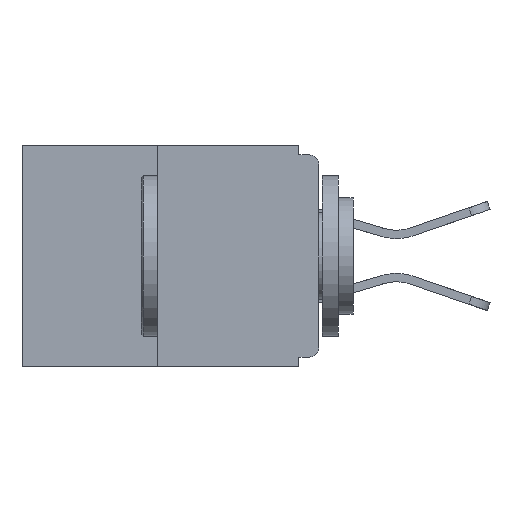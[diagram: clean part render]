
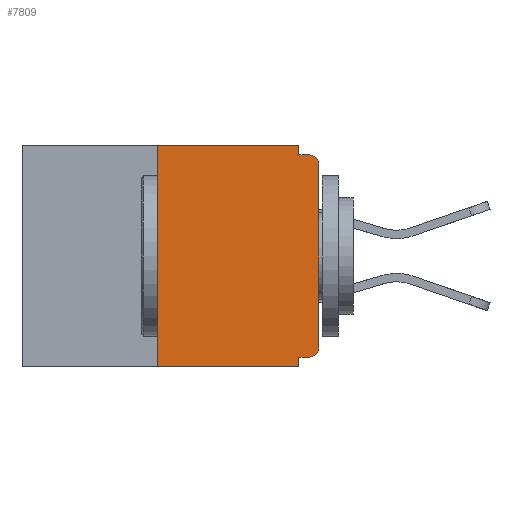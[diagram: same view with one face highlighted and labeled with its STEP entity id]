
A CAD part, left-side view. The second image highlights one B-rep face of the part: STEP entity #7809.
In plain terms, the highlighted planar face has unit normal (-1, 0, 0).
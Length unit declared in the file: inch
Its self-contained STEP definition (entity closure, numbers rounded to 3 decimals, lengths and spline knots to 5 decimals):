
#391 = DIRECTION ( 'NONE',  ( 0., -1., 0. ) ) ;
#411 = VECTOR ( 'NONE', #391, 39.37008 ) ;
#1763 = VERTEX_POINT ( 'NONE', #17021 ) ;
#2031 = CARTESIAN_POINT ( 'NONE',  ( 0., 0.015, -0.313 ) ) ;
#2103 = DIRECTION ( 'NONE',  ( 0., 0., 1. ) ) ;
#2507 = AXIS2_PLACEMENT_3D ( 'NONE', #2031, #16916, #10235 ) ;
#2935 = VERTEX_POINT ( 'NONE', #12909 ) ;
#2980 = CARTESIAN_POINT ( 'NONE',  ( 0., 0.031, -0.015 ) ) ;
#3116 = VECTOR ( 'NONE', #6594, 39.37008 ) ;
#3355 = EDGE_CURVE ( 'NONE', #2935, #6996, #9902, .T. ) ;
#3390 = VECTOR ( 'NONE', #12480, 39.37008 ) ;
#3739 = CARTESIAN_POINT ( 'NONE',  ( 0., 0.031, -0.343 ) ) ;
#3840 = CARTESIAN_POINT ( 'NONE',  ( 0., 0., 0. ) ) ;
#4443 = DIRECTION ( 'NONE',  ( 0., -1., 0. ) ) ;
#4661 = CARTESIAN_POINT ( 'NONE',  ( 0., 0.015, -0.03 ) ) ;
#4857 = AXIS2_PLACEMENT_3D ( 'NONE', #7709, #17078, #15802 ) ;
#4864 = CARTESIAN_POINT ( 'NONE',  ( 0., 0., -0.313 ) ) ;
#5045 = ORIENTED_EDGE ( 'NONE', *, *, #16976, .T. ) ;
#5208 = ORIENTED_EDGE ( 'NONE', *, *, #11124, .F. ) ;
#5465 = CARTESIAN_POINT ( 'NONE',  ( 0., 0.031, 0. ) ) ;
#5549 = VERTEX_POINT ( 'NONE', #4864 ) ;
#5625 = AXIS2_PLACEMENT_3D ( 'NONE', #4661, #9992, #8762 ) ;
#5684 = LINE ( 'NONE', #8951, #8833 ) ;
#5747 = CIRCLE ( 'NONE', #5625, 0.015 ) ;
#5835 = CARTESIAN_POINT ( 'NONE',  ( 0., 0.46, 0. ) ) ;
#5891 = CARTESIAN_POINT ( 'NONE',  ( 0., 0., -0.015 ) ) ;
#5989 = ORIENTED_EDGE ( 'NONE', *, *, #15294, .T. ) ;
#6482 = ORIENTED_EDGE ( 'NONE', *, *, #12952, .F. ) ;
#6594 = DIRECTION ( 'NONE',  ( 0., 0., -1. ) ) ;
#6836 = ORIENTED_EDGE ( 'NONE', *, *, #3355, .F. ) ;
#6996 = VERTEX_POINT ( 'NONE', #11893 ) ;
#7324 = VERTEX_POINT ( 'NONE', #11847 ) ;
#7512 = ORIENTED_EDGE ( 'NONE', *, *, #16741, .T. ) ;
#7709 = CARTESIAN_POINT ( 'NONE',  ( 0., 0.46, 0. ) ) ;
#7726 = VERTEX_POINT ( 'NONE', #14054 ) ;
#7809 = ADVANCED_FACE ( 'NONE', ( #8801 ), #14388, .F. ) ;
#8096 = VECTOR ( 'NONE', #4443, 39.37008 ) ;
#8340 = EDGE_CURVE ( 'NONE', #10479, #1763, #10663, .T. ) ;
#8451 = CARTESIAN_POINT ( 'NONE',  ( 0., 0.46, -0.343 ) ) ;
#8762 = DIRECTION ( 'NONE',  ( 0., 0., -1. ) ) ;
#8801 = FACE_OUTER_BOUND ( 'NONE', #10194, .T. ) ;
#8833 = VECTOR ( 'NONE', #12781, 39.37008 ) ;
#8951 = CARTESIAN_POINT ( 'NONE',  ( 0., 0., -0.328 ) ) ;
#9400 = ORIENTED_EDGE ( 'NONE', *, *, #8340, .F. ) ;
#9679 = CIRCLE ( 'NONE', #2507, 0.015 ) ;
#9817 = ORIENTED_EDGE ( 'NONE', *, *, #11422, .T. ) ;
#9902 = LINE ( 'NONE', #5835, #3390 ) ;
#9992 = DIRECTION ( 'NONE',  ( -1., 0., 0. ) ) ;
#10194 = EDGE_LOOP ( 'NONE', ( #6836, #5208, #7512, #9400, #12667, #5045, #9817, #5989, #6482, #14224 ) ) ;
#10235 = DIRECTION ( 'NONE',  ( 0., 0., -1. ) ) ;
#10479 = VERTEX_POINT ( 'NONE', #13318 ) ;
#10550 = VECTOR ( 'NONE', #13100, 39.37008 ) ;
#10663 = LINE ( 'NONE', #3739, #3116 ) ;
#10986 = VECTOR ( 'NONE', #2103, 39.37008 ) ;
#11124 = EDGE_CURVE ( 'NONE', #16109, #2935, #12472, .T. ) ;
#11422 = EDGE_CURVE ( 'NONE', #5549, #7726, #13708, .T. ) ;
#11847 = CARTESIAN_POINT ( 'NONE',  ( 0., 0.015, -0.328 ) ) ;
#11893 = CARTESIAN_POINT ( 'NONE',  ( 0., 0.031, 0. ) ) ;
#12183 = CARTESIAN_POINT ( 'NONE',  ( 0., 0.015, -0.015 ) ) ;
#12305 = LINE ( 'NONE', #5891, #8096 ) ;
#12472 = LINE ( 'NONE', #12854, #10986 ) ;
#12480 = DIRECTION ( 'NONE',  ( 0., -1., 0. ) ) ;
#12667 = ORIENTED_EDGE ( 'NONE', *, *, #16999, .F. ) ;
#12781 = DIRECTION ( 'NONE',  ( 0., 1., 0. ) ) ;
#12854 = CARTESIAN_POINT ( 'NONE',  ( 0., 0.25, 0. ) ) ;
#12909 = CARTESIAN_POINT ( 'NONE',  ( 0., 0.25, 0. ) ) ;
#12952 = EDGE_CURVE ( 'NONE', #13356, #13677, #12305, .T. ) ;
#13100 = DIRECTION ( 'NONE',  ( 0., 0., 1. ) ) ;
#13318 = CARTESIAN_POINT ( 'NONE',  ( 0., 0.031, -0.328 ) ) ;
#13356 = VERTEX_POINT ( 'NONE', #2980 ) ;
#13677 = VERTEX_POINT ( 'NONE', #12183 ) ;
#13708 = LINE ( 'NONE', #3840, #10550 ) ;
#14054 = CARTESIAN_POINT ( 'NONE',  ( 0., 0., -0.03 ) ) ;
#14224 = ORIENTED_EDGE ( 'NONE', *, *, #15774, .F. ) ;
#14388 = PLANE ( 'NONE',  #4857 ) ;
#14742 = LINE ( 'NONE', #5465, #15593 ) ;
#14847 = DIRECTION ( 'NONE',  ( 0., 0., -1. ) ) ;
#15294 = EDGE_CURVE ( 'NONE', #7726, #13677, #5747, .T. ) ;
#15593 = VECTOR ( 'NONE', #14847, 39.37008 ) ;
#15774 = EDGE_CURVE ( 'NONE', #6996, #13356, #14742, .T. ) ;
#15802 = DIRECTION ( 'NONE',  ( 0., 0., -1. ) ) ;
#16060 = CARTESIAN_POINT ( 'NONE',  ( 0., 0.25, -0.343 ) ) ;
#16109 = VERTEX_POINT ( 'NONE', #16060 ) ;
#16741 = EDGE_CURVE ( 'NONE', #16109, #1763, #16811, .T. ) ;
#16811 = LINE ( 'NONE', #8451, #411 ) ;
#16916 = DIRECTION ( 'NONE',  ( -1., 0., 0. ) ) ;
#16976 = EDGE_CURVE ( 'NONE', #7324, #5549, #9679, .T. ) ;
#16999 = EDGE_CURVE ( 'NONE', #7324, #10479, #5684, .T. ) ;
#17021 = CARTESIAN_POINT ( 'NONE',  ( 0., 0.031, -0.343 ) ) ;
#17078 = DIRECTION ( 'NONE',  ( 1., 0., 0. ) ) ;
